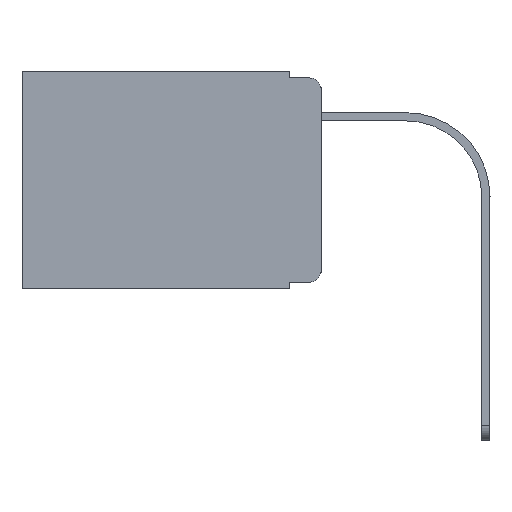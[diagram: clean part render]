
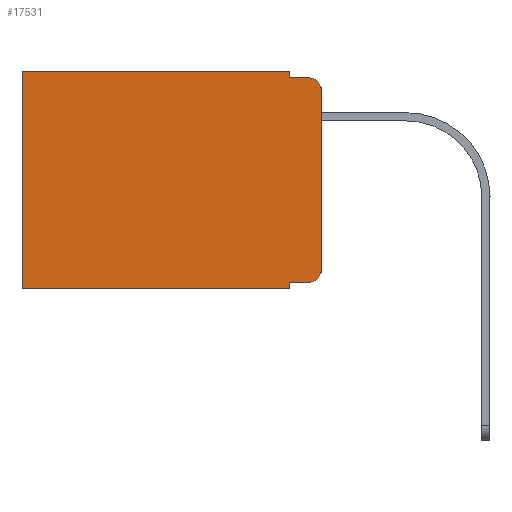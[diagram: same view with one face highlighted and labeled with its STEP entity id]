
A CAD part, left-side view. The second image highlights one B-rep face of the part: STEP entity #17531.
In plain terms, the highlighted planar face has unit normal (-1, 0, 0).
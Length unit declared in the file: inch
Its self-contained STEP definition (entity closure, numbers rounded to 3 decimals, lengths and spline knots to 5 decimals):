
#133 = CARTESIAN_POINT ( 'NONE',  ( 0.298, 0.051, -0.333 ) ) ;
#406 = DIRECTION ( 'NONE',  ( 0., 1., 0. ) ) ;
#431 = DIRECTION ( 'NONE',  ( 0., 0., -1. ) ) ;
#864 = VERTEX_POINT ( 'NONE', #9258 ) ;
#893 = VERTEX_POINT ( 'NONE', #3837 ) ;
#1223 = EDGE_CURVE ( 'NONE', #20864, #893, #9342, .T. ) ;
#1280 = PLANE ( 'NONE',  #12662 ) ;
#1496 = EDGE_CURVE ( 'NONE', #10793, #20864, #6584, .T. ) ;
#1520 = VERTEX_POINT ( 'NONE', #10252 ) ;
#2101 = EDGE_CURVE ( 'NONE', #10793, #14789, #14361, .T. ) ;
#2254 = CARTESIAN_POINT ( 'NONE',  ( 0.298, 0.02, -0.333 ) ) ;
#2352 = LINE ( 'NONE', #9359, #10313 ) ;
#2549 = CIRCLE ( 'NONE', #11020, 0.02 ) ;
#2765 = LINE ( 'NONE', #13492, #10696 ) ;
#2838 = EDGE_CURVE ( 'NONE', #864, #893, #15853, .T. ) ;
#2995 = VECTOR ( 'NONE', #14051, 39.37008 ) ;
#3532 = DIRECTION ( 'NONE',  ( 0., 0., -1. ) ) ;
#3837 = CARTESIAN_POINT ( 'NONE',  ( 0.298, 0.473, -0.343 ) ) ;
#3936 = CARTESIAN_POINT ( 'NONE',  ( 0.298, 0.051, 0. ) ) ;
#4557 = VERTEX_POINT ( 'NONE', #3936 ) ;
#4726 = AXIS2_PLACEMENT_3D ( 'NONE', #9776, #8308, #11982 ) ;
#4824 = FACE_OUTER_BOUND ( 'NONE', #13967, .T. ) ;
#5192 = EDGE_CURVE ( 'NONE', #4557, #864, #15396, .T. ) ;
#5322 = VECTOR ( 'NONE', #17142, 39.37008 ) ;
#5414 = CARTESIAN_POINT ( 'NONE',  ( 0.298, 0.051, -0.343 ) ) ;
#5538 = CARTESIAN_POINT ( 'NONE',  ( 0.298, 0.051, -0.333 ) ) ;
#5994 = EDGE_CURVE ( 'NONE', #4557, #18068, #2352, .T. ) ;
#6185 = DIRECTION ( 'NONE',  ( 0., 1., 0. ) ) ;
#6201 = DIRECTION ( 'NONE',  ( 0., 0., -1. ) ) ;
#6256 = ORIENTED_EDGE ( 'NONE', *, *, #8971, .T. ) ;
#6478 = EDGE_CURVE ( 'NONE', #18068, #16645, #2765, .T. ) ;
#6522 = CARTESIAN_POINT ( 'NONE',  ( 0.298, 0.02, -0.01 ) ) ;
#6584 = LINE ( 'NONE', #8751, #2995 ) ;
#6651 = VECTOR ( 'NONE', #10911, 39.37008 ) ;
#7088 = VECTOR ( 'NONE', #3532, 39.37008 ) ;
#7702 = VECTOR ( 'NONE', #6185, 39.37008 ) ;
#7925 = ORIENTED_EDGE ( 'NONE', *, *, #1496, .F. ) ;
#8059 = CARTESIAN_POINT ( 'NONE',  ( 0.298, 0., 0. ) ) ;
#8308 = DIRECTION ( 'NONE',  ( -1., 0., 0. ) ) ;
#8751 = CARTESIAN_POINT ( 'NONE',  ( 0.298, 0.051, 0. ) ) ;
#8971 = EDGE_CURVE ( 'NONE', #1520, #16645, #10249, .T. ) ;
#9258 = CARTESIAN_POINT ( 'NONE',  ( 0.298, 0.473, 0. ) ) ;
#9342 = LINE ( 'NONE', #11196, #13638 ) ;
#9359 = CARTESIAN_POINT ( 'NONE',  ( 0.298, 0.051, 0. ) ) ;
#9695 = DIRECTION ( 'NONE',  ( -1., 0., 0. ) ) ;
#9758 = CARTESIAN_POINT ( 'NONE',  ( 0.298, 0., 0. ) ) ;
#9776 = CARTESIAN_POINT ( 'NONE',  ( 0.298, 0.02, -0.03 ) ) ;
#10086 = ORIENTED_EDGE ( 'NONE', *, *, #2101, .T. ) ;
#10150 = ORIENTED_EDGE ( 'NONE', *, *, #13498, .T. ) ;
#10211 = ORIENTED_EDGE ( 'NONE', *, *, #2838, .T. ) ;
#10249 = CIRCLE ( 'NONE', #4726, 0.02 ) ;
#10252 = CARTESIAN_POINT ( 'NONE',  ( 0.298, 0., -0.03 ) ) ;
#10313 = VECTOR ( 'NONE', #431, 39.37008 ) ;
#10316 = CARTESIAN_POINT ( 'NONE',  ( 0.298, 0., -0.313 ) ) ;
#10696 = VECTOR ( 'NONE', #11418, 39.37008 ) ;
#10793 = VERTEX_POINT ( 'NONE', #5538 ) ;
#10911 = DIRECTION ( 'NONE',  ( 0., -1., 0. ) ) ;
#11020 = AXIS2_PLACEMENT_3D ( 'NONE', #16973, #9695, #11544 ) ;
#11196 = CARTESIAN_POINT ( 'NONE',  ( 0.298, 0., -0.343 ) ) ;
#11418 = DIRECTION ( 'NONE',  ( 0., -1., 0. ) ) ;
#11544 = DIRECTION ( 'NONE',  ( 0., 0., -1. ) ) ;
#11982 = DIRECTION ( 'NONE',  ( 0., 0., -1. ) ) ;
#12662 = AXIS2_PLACEMENT_3D ( 'NONE', #8059, #17048, #6201 ) ;
#13248 = VERTEX_POINT ( 'NONE', #10316 ) ;
#13492 = CARTESIAN_POINT ( 'NONE',  ( 0.298, 0.051, -0.01 ) ) ;
#13498 = EDGE_CURVE ( 'NONE', #14789, #13248, #2549, .T. ) ;
#13638 = VECTOR ( 'NONE', #406, 39.37008 ) ;
#13967 = EDGE_LOOP ( 'NONE', ( #20679, #6256, #21616, #14286, #18076, #10211, #17397, #7925, #10086, #10150 ) ) ;
#14051 = DIRECTION ( 'NONE',  ( 0., 0., -1. ) ) ;
#14163 = EDGE_CURVE ( 'NONE', #1520, #13248, #15987, .T. ) ;
#14286 = ORIENTED_EDGE ( 'NONE', *, *, #5994, .F. ) ;
#14361 = LINE ( 'NONE', #133, #6651 ) ;
#14789 = VERTEX_POINT ( 'NONE', #2254 ) ;
#15396 = LINE ( 'NONE', #9758, #7702 ) ;
#15853 = LINE ( 'NONE', #19155, #5322 ) ;
#15987 = LINE ( 'NONE', #19623, #7088 ) ;
#16645 = VERTEX_POINT ( 'NONE', #6522 ) ;
#16973 = CARTESIAN_POINT ( 'NONE',  ( 0.298, 0.02, -0.313 ) ) ;
#17048 = DIRECTION ( 'NONE',  ( 1., 0., 0. ) ) ;
#17142 = DIRECTION ( 'NONE',  ( 0., 0., -1. ) ) ;
#17397 = ORIENTED_EDGE ( 'NONE', *, *, #1223, .F. ) ;
#17531 = ADVANCED_FACE ( 'NONE', ( #4824 ), #1280, .F. ) ;
#18068 = VERTEX_POINT ( 'NONE', #20399 ) ;
#18076 = ORIENTED_EDGE ( 'NONE', *, *, #5192, .T. ) ;
#19155 = CARTESIAN_POINT ( 'NONE',  ( 0.298, 0.473, 0. ) ) ;
#19623 = CARTESIAN_POINT ( 'NONE',  ( 0.298, 0., 0. ) ) ;
#20399 = CARTESIAN_POINT ( 'NONE',  ( 0.298, 0.051, -0.01 ) ) ;
#20679 = ORIENTED_EDGE ( 'NONE', *, *, #14163, .F. ) ;
#20864 = VERTEX_POINT ( 'NONE', #5414 ) ;
#21616 = ORIENTED_EDGE ( 'NONE', *, *, #6478, .F. ) ;
